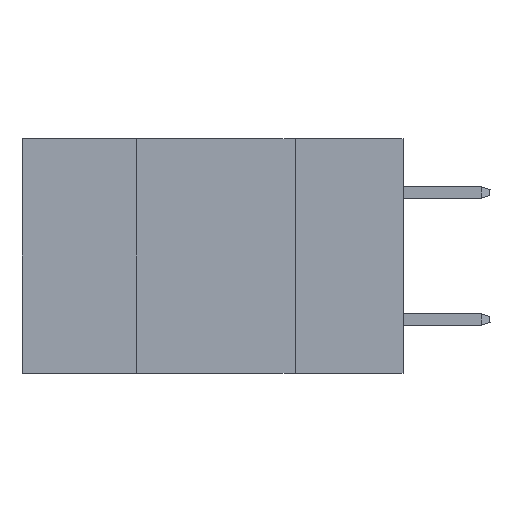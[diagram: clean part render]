
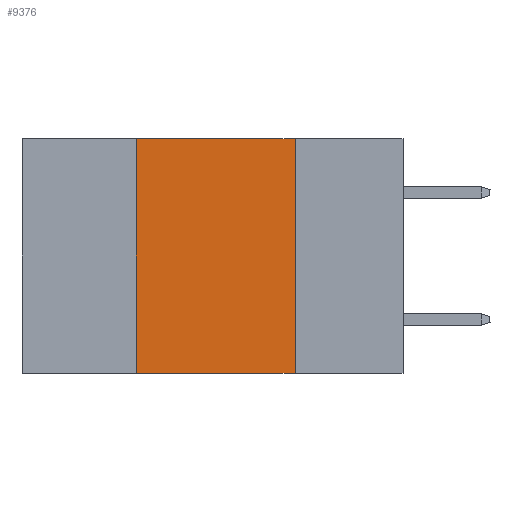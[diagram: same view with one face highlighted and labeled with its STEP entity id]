
A CAD part, left-side view. The second image highlights one B-rep face of the part: STEP entity #9376.
In plain terms, the highlighted planar face has unit normal (-1, 0, 0).
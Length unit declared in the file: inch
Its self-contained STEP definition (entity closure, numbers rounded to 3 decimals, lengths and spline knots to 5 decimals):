
#580 = ORIENTED_EDGE ( 'NONE', *, *, #14925, .F. ) ;
#1294 = LINE ( 'NONE', #6714, #9107 ) ;
#1392 = CARTESIAN_POINT ( 'NONE',  ( 0., 0.17, -0.37 ) ) ;
#1399 = CARTESIAN_POINT ( 'NONE',  ( 0., 0.17, 0. ) ) ;
#1563 = CARTESIAN_POINT ( 'NONE',  ( 0., 0.42, 0. ) ) ;
#1920 = VERTEX_POINT ( 'NONE', #11958 ) ;
#2120 = AXIS2_PLACEMENT_3D ( 'NONE', #15254, #7297, #7045 ) ;
#2357 = LINE ( 'NONE', #9038, #6918 ) ;
#3190 = EDGE_CURVE ( 'NONE', #8329, #8705, #13952, .T. ) ;
#4092 = VECTOR ( 'NONE', #8606, 39.37008 ) ;
#4413 = DIRECTION ( 'NONE',  ( 0., -1., 0. ) ) ;
#4837 = EDGE_LOOP ( 'NONE', ( #16037, #10976, #580, #9486 ) ) ;
#5635 = VERTEX_POINT ( 'NONE', #13261 ) ;
#6714 = CARTESIAN_POINT ( 'NONE',  ( 0., 0.6, 0. ) ) ;
#6792 = DIRECTION ( 'NONE',  ( 0., 0., 1. ) ) ;
#6918 = VECTOR ( 'NONE', #7686, 39.37008 ) ;
#7045 = DIRECTION ( 'NONE',  ( 0., 0., -1. ) ) ;
#7297 = DIRECTION ( 'NONE',  ( 1., 0., 0. ) ) ;
#7686 = DIRECTION ( 'NONE',  ( 0., -1., 0. ) ) ;
#8329 = VERTEX_POINT ( 'NONE', #1399 ) ;
#8606 = DIRECTION ( 'NONE',  ( 0., 0., -1. ) ) ;
#8705 = VERTEX_POINT ( 'NONE', #1392 ) ;
#8783 = CARTESIAN_POINT ( 'NONE',  ( 0., 0.17, 0. ) ) ;
#9038 = CARTESIAN_POINT ( 'NONE',  ( 0., 0.6, -0.37 ) ) ;
#9107 = VECTOR ( 'NONE', #4413, 39.37008 ) ;
#9255 = EDGE_CURVE ( 'NONE', #1920, #8705, #2357, .T. ) ;
#9376 = ADVANCED_FACE ( 'NONE', ( #9733 ), #12222, .F. ) ;
#9462 = LINE ( 'NONE', #1563, #13311 ) ;
#9486 = ORIENTED_EDGE ( 'NONE', *, *, #9255, .T. ) ;
#9733 = FACE_OUTER_BOUND ( 'NONE', #4837, .T. ) ;
#10976 = ORIENTED_EDGE ( 'NONE', *, *, #15890, .F. ) ;
#11958 = CARTESIAN_POINT ( 'NONE',  ( 0., 0.42, -0.37 ) ) ;
#12222 = PLANE ( 'NONE',  #2120 ) ;
#13261 = CARTESIAN_POINT ( 'NONE',  ( 0., 0.42, 0. ) ) ;
#13311 = VECTOR ( 'NONE', #6792, 39.37008 ) ;
#13952 = LINE ( 'NONE', #8783, #4092 ) ;
#14925 = EDGE_CURVE ( 'NONE', #1920, #5635, #9462, .T. ) ;
#15254 = CARTESIAN_POINT ( 'NONE',  ( 0., 0.6, 0. ) ) ;
#15890 = EDGE_CURVE ( 'NONE', #5635, #8329, #1294, .T. ) ;
#16037 = ORIENTED_EDGE ( 'NONE', *, *, #3190, .F. ) ;
